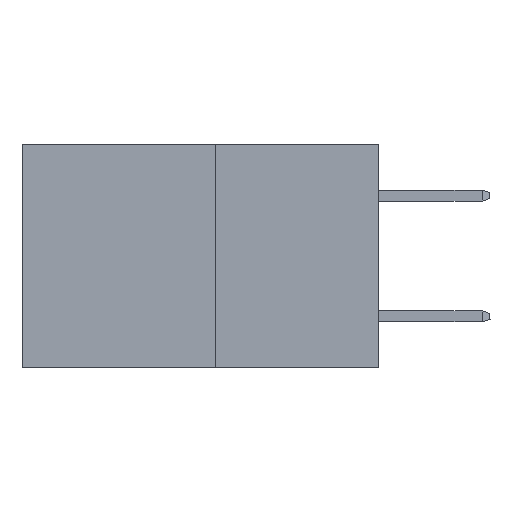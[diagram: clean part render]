
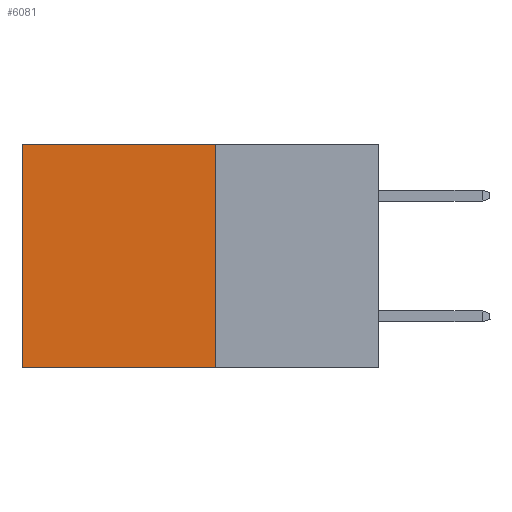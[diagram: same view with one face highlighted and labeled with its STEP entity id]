
A CAD part, left-side view. The second image highlights one B-rep face of the part: STEP entity #6081.
In plain terms, the highlighted planar face has unit normal (-1, 0, 0).
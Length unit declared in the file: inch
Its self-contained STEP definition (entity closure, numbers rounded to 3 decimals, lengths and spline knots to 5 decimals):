
#257 = EDGE_CURVE ( 'NONE', #4167, #14147, #7436, .T. ) ;
#406 = DIRECTION ( 'NONE',  ( 0., 0., -1. ) ) ;
#488 = VECTOR ( 'NONE', #10431, 39.37008 ) ;
#926 = ORIENTED_EDGE ( 'NONE', *, *, #10962, .F. ) ;
#992 = CARTESIAN_POINT ( 'NONE',  ( 0.277, 0.27, -0.37 ) ) ;
#1151 = EDGE_CURVE ( 'NONE', #10123, #9047, #3323, .T. ) ;
#1573 = VECTOR ( 'NONE', #8517, 39.37008 ) ;
#2019 = PLANE ( 'NONE',  #5652 ) ;
#2834 = ORIENTED_EDGE ( 'NONE', *, *, #1151, .F. ) ;
#2867 = ORIENTED_EDGE ( 'NONE', *, *, #257, .T. ) ;
#3267 = DIRECTION ( 'NONE',  ( 1., 0., 0. ) ) ;
#3323 = LINE ( 'NONE', #3967, #12804 ) ;
#3836 = VECTOR ( 'NONE', #10936, 39.37008 ) ;
#3967 = CARTESIAN_POINT ( 'NONE',  ( 0.277, 0.27, -0.37 ) ) ;
#4167 = VERTEX_POINT ( 'NONE', #9349 ) ;
#5652 = AXIS2_PLACEMENT_3D ( 'NONE', #9410, #3267, #11925 ) ;
#6081 = ADVANCED_FACE ( 'NONE', ( #7680 ), #2019, .F. ) ;
#6654 = CARTESIAN_POINT ( 'NONE',  ( 0.277, 0.59, -0.37 ) ) ;
#6727 = CARTESIAN_POINT ( 'NONE',  ( 0.277, 0.27, 0. ) ) ;
#7155 = LINE ( 'NONE', #6727, #488 ) ;
#7164 = LINE ( 'NONE', #992, #3836 ) ;
#7436 = LINE ( 'NONE', #14434, #1573 ) ;
#7680 = FACE_OUTER_BOUND ( 'NONE', #9711, .T. ) ;
#8265 = CARTESIAN_POINT ( 'NONE',  ( 0.277, 0.27, 0. ) ) ;
#8517 = DIRECTION ( 'NONE',  ( 0., 0., -1. ) ) ;
#9047 = VERTEX_POINT ( 'NONE', #10204 ) ;
#9349 = CARTESIAN_POINT ( 'NONE',  ( 0.277, 0.59, 0. ) ) ;
#9410 = CARTESIAN_POINT ( 'NONE',  ( 0.277, 0.27, -0.37 ) ) ;
#9711 = EDGE_LOOP ( 'NONE', ( #2867, #926, #2834, #11599 ) ) ;
#10123 = VERTEX_POINT ( 'NONE', #8265 ) ;
#10204 = CARTESIAN_POINT ( 'NONE',  ( 0.277, 0.27, -0.37 ) ) ;
#10431 = DIRECTION ( 'NONE',  ( 0., 1., 0. ) ) ;
#10936 = DIRECTION ( 'NONE',  ( 0., 1., 0. ) ) ;
#10962 = EDGE_CURVE ( 'NONE', #9047, #14147, #7164, .T. ) ;
#11599 = ORIENTED_EDGE ( 'NONE', *, *, #11951, .T. ) ;
#11925 = DIRECTION ( 'NONE',  ( 0., 0., -1. ) ) ;
#11951 = EDGE_CURVE ( 'NONE', #10123, #4167, #7155, .T. ) ;
#12804 = VECTOR ( 'NONE', #406, 39.37008 ) ;
#14147 = VERTEX_POINT ( 'NONE', #6654 ) ;
#14434 = CARTESIAN_POINT ( 'NONE',  ( 0.277, 0.59, -0.37 ) ) ;
